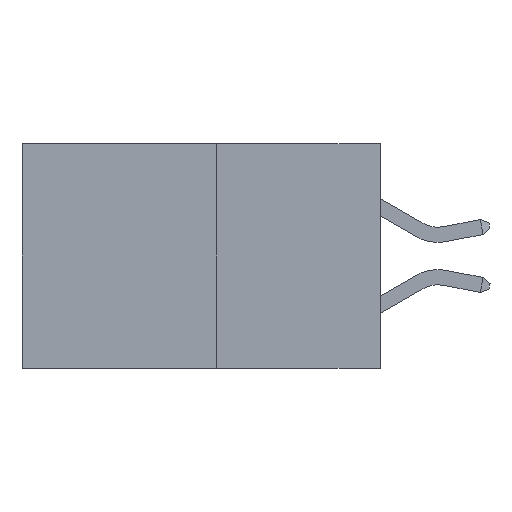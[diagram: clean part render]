
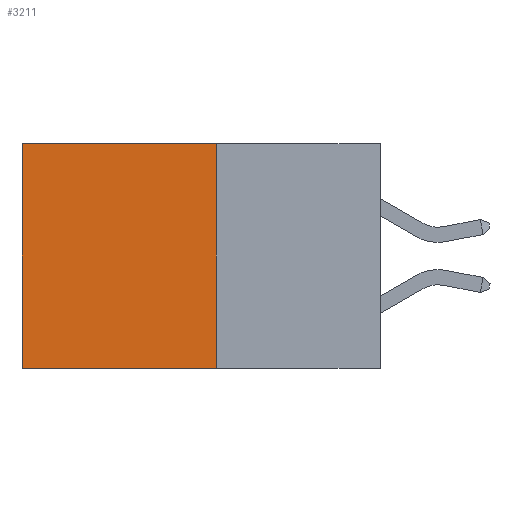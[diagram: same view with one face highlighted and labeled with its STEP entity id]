
A CAD part, left-side view. The second image highlights one B-rep face of the part: STEP entity #3211.
In plain terms, the highlighted planar face has unit normal (-1, 0, 0).
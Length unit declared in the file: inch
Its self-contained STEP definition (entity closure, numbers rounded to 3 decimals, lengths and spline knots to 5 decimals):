
#353 = ORIENTED_EDGE ( 'NONE', *, *, #371, .T. ) ;
#371 = EDGE_CURVE ( 'NONE', #3122, #4678, #1033, .T. ) ;
#593 = VECTOR ( 'NONE', #10665, 39.37008 ) ;
#829 = VERTEX_POINT ( 'NONE', #12225 ) ;
#865 = VERTEX_POINT ( 'NONE', #4675 ) ;
#1033 = LINE ( 'NONE', #7519, #593 ) ;
#1638 = CARTESIAN_POINT ( 'NONE',  ( 0.277, 0.59, -0.37 ) ) ;
#1778 = EDGE_CURVE ( 'NONE', #865, #4678, #4182, .T. ) ;
#2445 = ORIENTED_EDGE ( 'NONE', *, *, #11098, .F. ) ;
#3122 = VERTEX_POINT ( 'NONE', #11996 ) ;
#3211 = ADVANCED_FACE ( 'NONE', ( #13092 ), #8251, .F. ) ;
#3522 = ORIENTED_EDGE ( 'NONE', *, *, #7819, .T. ) ;
#4182 = LINE ( 'NONE', #6956, #12617 ) ;
#4675 = CARTESIAN_POINT ( 'NONE',  ( 0.277, 0.27, -0.37 ) ) ;
#4678 = VERTEX_POINT ( 'NONE', #1638 ) ;
#5941 = AXIS2_PLACEMENT_3D ( 'NONE', #8834, #8466, #8460 ) ;
#6956 = CARTESIAN_POINT ( 'NONE',  ( 0.277, 0.27, -0.37 ) ) ;
#7319 = CARTESIAN_POINT ( 'NONE',  ( 0.277, 0.27, -0.37 ) ) ;
#7340 = DIRECTION ( 'NONE',  ( 0., 0., -1. ) ) ;
#7519 = CARTESIAN_POINT ( 'NONE',  ( 0.277, 0.59, -0.37 ) ) ;
#7819 = EDGE_CURVE ( 'NONE', #829, #3122, #8010, .T. ) ;
#8010 = LINE ( 'NONE', #10103, #13729 ) ;
#8251 = PLANE ( 'NONE',  #5941 ) ;
#8460 = DIRECTION ( 'NONE',  ( 0., 0., -1. ) ) ;
#8466 = DIRECTION ( 'NONE',  ( 1., 0., 0. ) ) ;
#8690 = EDGE_LOOP ( 'NONE', ( #353, #8892, #2445, #3522 ) ) ;
#8724 = VECTOR ( 'NONE', #7340, 39.37008 ) ;
#8834 = CARTESIAN_POINT ( 'NONE',  ( 0.277, 0.27, -0.37 ) ) ;
#8892 = ORIENTED_EDGE ( 'NONE', *, *, #1778, .F. ) ;
#9724 = DIRECTION ( 'NONE',  ( 0., 1., 0. ) ) ;
#9987 = DIRECTION ( 'NONE',  ( 0., 1., 0. ) ) ;
#10103 = CARTESIAN_POINT ( 'NONE',  ( 0.277, 0.27, 0. ) ) ;
#10665 = DIRECTION ( 'NONE',  ( 0., 0., -1. ) ) ;
#11098 = EDGE_CURVE ( 'NONE', #829, #865, #11652, .T. ) ;
#11652 = LINE ( 'NONE', #7319, #8724 ) ;
#11996 = CARTESIAN_POINT ( 'NONE',  ( 0.277, 0.59, 0. ) ) ;
#12225 = CARTESIAN_POINT ( 'NONE',  ( 0.277, 0.27, 0. ) ) ;
#12617 = VECTOR ( 'NONE', #9724, 39.37008 ) ;
#13092 = FACE_OUTER_BOUND ( 'NONE', #8690, .T. ) ;
#13729 = VECTOR ( 'NONE', #9987, 39.37008 ) ;
